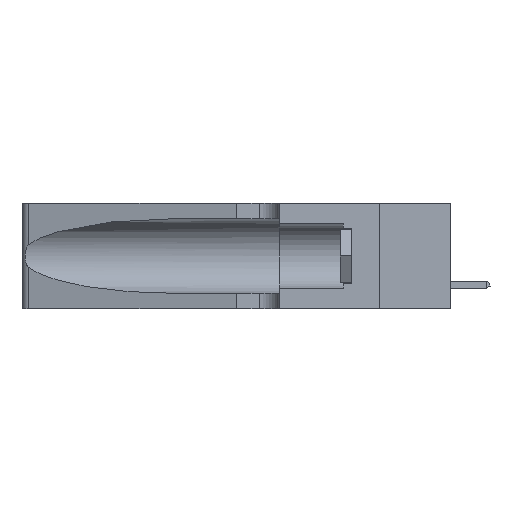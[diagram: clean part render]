
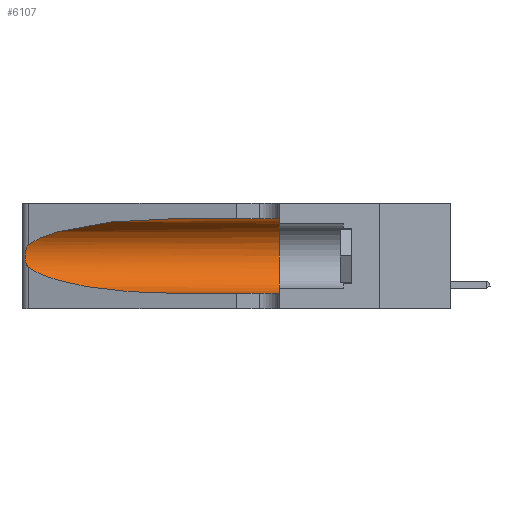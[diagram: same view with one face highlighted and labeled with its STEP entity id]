
A CAD part, left-side view. The second image highlights one B-rep face of the part: STEP entity #6107.
In plain terms, the highlighted cylindrical face has radius 3.308 mm (diameter 6.617 mm), a partial arc.
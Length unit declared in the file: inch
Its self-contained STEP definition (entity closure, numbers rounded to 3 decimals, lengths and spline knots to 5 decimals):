
#1272 = CARTESIAN_POINT ( 'NONE',  ( 0.25787, 1.23484, 0.2124 ) ) ;
#1410 = VERTEX_POINT ( 'NONE', #32437 ) ;
#2271 = CARTESIAN_POINT ( 'NONE',  ( 0.25555, 1.22993, 0.14849 ) ) ;
#3100 = AXIS2_PLACEMENT_3D ( 'NONE', #15705, #19523, #26820 ) ;
#3729 = EDGE_CURVE ( 'NONE', #36377, #15222, #37813, .T. ) ;
#4853 = CARTESIAN_POINT ( 'NONE',  ( 0.25854, 1.2359, 0.20912 ) ) ;
#5010 = CARTESIAN_POINT ( 'NONE',  ( 0.25856, 1.23593, 0.16098 ) ) ;
#5633 = VECTOR ( 'NONE', #41403, 39.37008 ) ;
#6107 = ADVANCED_FACE ( 'NONE', ( #27788 ), #45605, .F. ) ;
#8719 = ORIENTED_EDGE ( 'NONE', *, *, #13934, .T. ) ;
#8817 = B_SPLINE_CURVE_WITH_KNOTS ( 'NONE', 3,
 ( #30644, #19056, #26680, #1272, #4853, #37715, #19558, #45133, #26850, #5010, #30485, #30965, #2271, #27629 ),
 .UNSPECIFIED., .F., .F.,
 ( 4, 2, 2, 2, 2, 2, 4 ),
 ( 0., 0.00027, 0.00053, 0.00107, 0.0016, 0.00187, 0.00214 ),
 .UNSPECIFIED. ) ;
#9048 = LINE ( 'NONE', #34917, #5633 ) ;
#9341 = CIRCLE ( 'NONE', #24670, 0.13025 ) ;
#9539 = CARTESIAN_POINT ( 'NONE',  ( 0.1305, 0.35, 0.185 ) ) ;
#10203 = ORIENTED_EDGE ( 'NONE', *, *, #16527, .T. ) ;
#11933 = CARTESIAN_POINT ( 'NONE',  ( 0.2373, 1.15595, 0.08982 ) ) ;
#12647 = CARTESIAN_POINT ( 'NONE',  ( 0.2373, 1.15595, 0.28018 ) ) ;
#13034 = ORIENTED_EDGE ( 'NONE', *, *, #44682, .T. ) ;
#13934 = EDGE_CURVE ( 'NONE', #33718, #1410, #9048, .T. ) ;
#14708 =( BOUNDED_CURVE ( )  B_SPLINE_CURVE ( 3, ( #26738, #11933, #22947, #44542 ),
 .UNSPECIFIED., .F., .F. ) 
 B_SPLINE_CURVE_WITH_KNOTS ( ( 4, 4 ),
 ( 3.44316, 4.71239 ),
 .UNSPECIFIED. ) 
 CURVE ( )  GEOMETRIC_REPRESENTATION_ITEM ( )  RATIONAL_B_SPLINE_CURVE ( ( 1., 0.87, 0.87, 1. ) ) 
 REPRESENTATION_ITEM ( '' )  );
#15156 = CARTESIAN_POINT ( 'NONE',  ( 0.1305, 1.61858, 0.31525 ) ) ;
#15222 = VERTEX_POINT ( 'NONE', #24573 ) ;
#15705 = CARTESIAN_POINT ( 'NONE',  ( 0.1305, 1.61858, 0.185 ) ) ;
#16146 = VECTOR ( 'NONE', #22481, 39.37008 ) ;
#16527 = EDGE_CURVE ( 'NONE', #38953, #18228, #8817, .T. ) ;
#18228 = VERTEX_POINT ( 'NONE', #45374 ) ;
#19056 = CARTESIAN_POINT ( 'NONE',  ( 0.25555, 1.22994, 0.2215 ) ) ;
#19523 = DIRECTION ( 'NONE',  ( 0., -1., 0. ) ) ;
#19558 = CARTESIAN_POINT ( 'NONE',  ( 0.26075, 1.23896, 0.19203 ) ) ;
#19670 = CARTESIAN_POINT ( 'NONE',  ( 0.1305, 0.72297, 0.31525 ) ) ;
#21736 = EDGE_LOOP ( 'NONE', ( #29891, #10203, #13034, #8719, #22934, #23143 ) ) ;
#22020 = EDGE_CURVE ( 'NONE', #15222, #1410, #9341, .T. ) ;
#22481 = DIRECTION ( 'NONE',  ( 0., -1., 0. ) ) ;
#22934 = ORIENTED_EDGE ( 'NONE', *, *, #22020, .F. ) ;
#22947 = CARTESIAN_POINT ( 'NONE',  ( 0.18966, 0.96281, 0.05475 ) ) ;
#23143 = ORIENTED_EDGE ( 'NONE', *, *, #3729, .F. ) ;
#24573 = CARTESIAN_POINT ( 'NONE',  ( 0.1305, 0.35, 0.31525 ) ) ;
#24670 = AXIS2_PLACEMENT_3D ( 'NONE', #9539, #31546, #38771 ) ;
#26680 = CARTESIAN_POINT ( 'NONE',  ( 0.25639, 1.23184, 0.21858 ) ) ;
#26738 = CARTESIAN_POINT ( 'NONE',  ( 0.25487, 1.22718, 0.14631 ) ) ;
#26820 = DIRECTION ( 'NONE',  ( 0., 0., -1. ) ) ;
#26850 = CARTESIAN_POINT ( 'NONE',  ( 0.26017, 1.23833, 0.17102 ) ) ;
#27109 = CARTESIAN_POINT ( 'NONE',  ( 0.18966, 0.96281, 0.31525 ) ) ;
#27629 = CARTESIAN_POINT ( 'NONE',  ( 0.25487, 1.22718, 0.14631 ) ) ;
#27788 = FACE_OUTER_BOUND ( 'NONE', #21736, .T. ) ;
#29891 = ORIENTED_EDGE ( 'NONE', *, *, #32402, .T. ) ;
#30485 = CARTESIAN_POINT ( 'NONE',  ( 0.25789, 1.23486, 0.15765 ) ) ;
#30644 = CARTESIAN_POINT ( 'NONE',  ( 0.25487, 1.22718, 0.22369 ) ) ;
#30965 = CARTESIAN_POINT ( 'NONE',  ( 0.25639, 1.23186, 0.15144 ) ) ;
#31546 = DIRECTION ( 'NONE',  ( 0., 1., 0. ) ) ;
#32297 = CARTESIAN_POINT ( 'NONE',  ( 0.1305, 0.72297, 0.05475 ) ) ;
#32402 = EDGE_CURVE ( 'NONE', #36377, #38953, #33627, .T. ) ;
#32437 = CARTESIAN_POINT ( 'NONE',  ( 0.1305, 0.35, 0.05475 ) ) ;
#33627 =( BOUNDED_CURVE ( )  B_SPLINE_CURVE ( 3, ( #19670, #27109, #12647, #45570 ),
 .UNSPECIFIED., .F., .F. ) 
 B_SPLINE_CURVE_WITH_KNOTS ( ( 4, 4 ),
 ( 1.5708, 2.84003 ),
 .UNSPECIFIED. ) 
 CURVE ( )  GEOMETRIC_REPRESENTATION_ITEM ( )  RATIONAL_B_SPLINE_CURVE ( ( 1., 0.87, 0.87, 1. ) ) 
 REPRESENTATION_ITEM ( '' )  );
#33718 = VERTEX_POINT ( 'NONE', #32297 ) ;
#34917 = CARTESIAN_POINT ( 'NONE',  ( 0.1305, 1.61858, 0.05475 ) ) ;
#36377 = VERTEX_POINT ( 'NONE', #41533 ) ;
#37715 = CARTESIAN_POINT ( 'NONE',  ( 0.26018, 1.23835, 0.19895 ) ) ;
#37813 = LINE ( 'NONE', #15156, #16146 ) ;
#38771 = DIRECTION ( 'NONE',  ( 0., 0., 1. ) ) ;
#38953 = VERTEX_POINT ( 'NONE', #44030 ) ;
#41403 = DIRECTION ( 'NONE',  ( 0., -1., 0. ) ) ;
#41533 = CARTESIAN_POINT ( 'NONE',  ( 0.1305, 0.72297, 0.31525 ) ) ;
#44030 = CARTESIAN_POINT ( 'NONE',  ( 0.25487, 1.22718, 0.22369 ) ) ;
#44542 = CARTESIAN_POINT ( 'NONE',  ( 0.1305, 0.72297, 0.05475 ) ) ;
#44682 = EDGE_CURVE ( 'NONE', #18228, #33718, #14708, .T. ) ;
#45133 = CARTESIAN_POINT ( 'NONE',  ( 0.26075, 1.23896, 0.178 ) ) ;
#45374 = CARTESIAN_POINT ( 'NONE',  ( 0.25487, 1.22718, 0.14631 ) ) ;
#45570 = CARTESIAN_POINT ( 'NONE',  ( 0.25487, 1.22718, 0.22369 ) ) ;
#45605 = CYLINDRICAL_SURFACE ( 'NONE', #3100, 0.13025 ) ;
